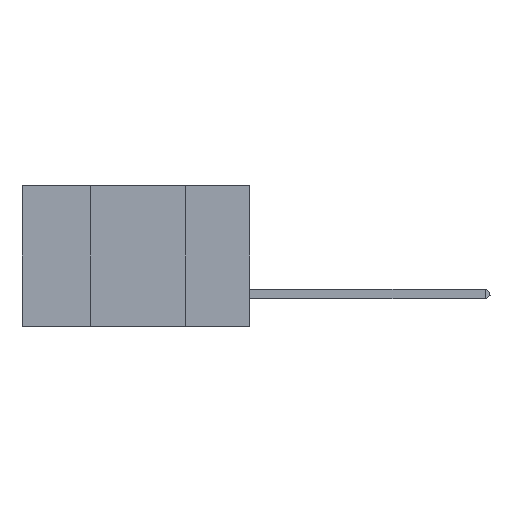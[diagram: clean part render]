
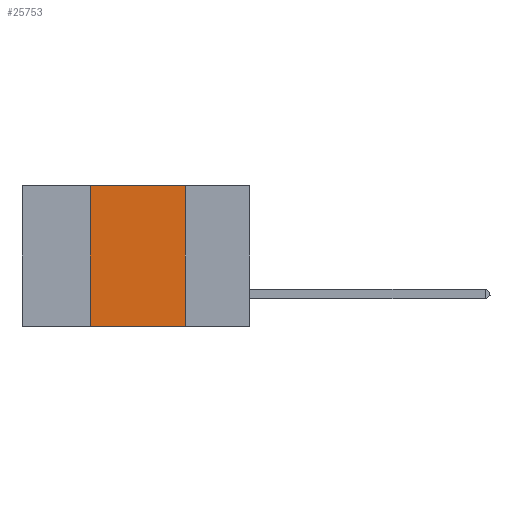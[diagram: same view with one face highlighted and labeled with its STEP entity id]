
A CAD part, left-side view. The second image highlights one B-rep face of the part: STEP entity #25753.
In plain terms, the highlighted planar face has unit normal (-1, 0, 0).
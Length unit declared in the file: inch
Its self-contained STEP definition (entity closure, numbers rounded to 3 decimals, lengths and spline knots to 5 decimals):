
#1418 = EDGE_CURVE ( 'NONE', #3385, #23163, #42534, .T. ) ;
#3233 = CARTESIAN_POINT ( 'NONE',  ( 0., 0.6, 0. ) ) ;
#3385 = VERTEX_POINT ( 'NONE', #21067 ) ;
#5198 = VECTOR ( 'NONE', #25023, 39.37008 ) ;
#10373 = CARTESIAN_POINT ( 'NONE',  ( 0., 0.42, 0. ) ) ;
#11152 = CARTESIAN_POINT ( 'NONE',  ( 0., 0.17, 0. ) ) ;
#11184 = DIRECTION ( 'NONE',  ( 1., 0., 0. ) ) ;
#11407 = DIRECTION ( 'NONE',  ( 0., -1., 0. ) ) ;
#11448 = EDGE_CURVE ( 'NONE', #3385, #27252, #18454, .T. ) ;
#14592 = VERTEX_POINT ( 'NONE', #30321 ) ;
#17921 = EDGE_CURVE ( 'NONE', #14592, #27252, #38860, .T. ) ;
#18454 = LINE ( 'NONE', #43572, #39478 ) ;
#18485 = VECTOR ( 'NONE', #31885, 39.37008 ) ;
#21067 = CARTESIAN_POINT ( 'NONE',  ( 0., 0.42, -0.37 ) ) ;
#21617 = EDGE_CURVE ( 'NONE', #23163, #14592, #35410, .T. ) ;
#23163 = VERTEX_POINT ( 'NONE', #23632 ) ;
#23632 = CARTESIAN_POINT ( 'NONE',  ( 0., 0.42, 0. ) ) ;
#24274 = ORIENTED_EDGE ( 'NONE', *, *, #17921, .F. ) ;
#24692 = DIRECTION ( 'NONE',  ( 0., 0., 1. ) ) ;
#25023 = DIRECTION ( 'NONE',  ( 0., 0., -1. ) ) ;
#25753 = ADVANCED_FACE ( 'NONE', ( #29034 ), #43342, .F. ) ;
#26453 = EDGE_LOOP ( 'NONE', ( #24274, #34788, #36352, #30026 ) ) ;
#27252 = VERTEX_POINT ( 'NONE', #38622 ) ;
#29034 = FACE_OUTER_BOUND ( 'NONE', #26453, .T. ) ;
#30026 = ORIENTED_EDGE ( 'NONE', *, *, #11448, .T. ) ;
#30321 = CARTESIAN_POINT ( 'NONE',  ( 0., 0.17, 0. ) ) ;
#30773 = VECTOR ( 'NONE', #24692, 39.37008 ) ;
#31885 = DIRECTION ( 'NONE',  ( 0., -1., 0. ) ) ;
#33019 = DIRECTION ( 'NONE',  ( 0., 0., -1. ) ) ;
#33254 = CARTESIAN_POINT ( 'NONE',  ( 0., 0.6, 0. ) ) ;
#34788 = ORIENTED_EDGE ( 'NONE', *, *, #21617, .F. ) ;
#35410 = LINE ( 'NONE', #3233, #18485 ) ;
#36352 = ORIENTED_EDGE ( 'NONE', *, *, #1418, .F. ) ;
#38622 = CARTESIAN_POINT ( 'NONE',  ( 0., 0.17, -0.37 ) ) ;
#38860 = LINE ( 'NONE', #11152, #5198 ) ;
#39478 = VECTOR ( 'NONE', #11407, 39.37008 ) ;
#42534 = LINE ( 'NONE', #10373, #30773 ) ;
#43342 = PLANE ( 'NONE',  #45596 ) ;
#43572 = CARTESIAN_POINT ( 'NONE',  ( 0., 0.6, -0.37 ) ) ;
#45596 = AXIS2_PLACEMENT_3D ( 'NONE', #33254, #11184, #33019 ) ;
